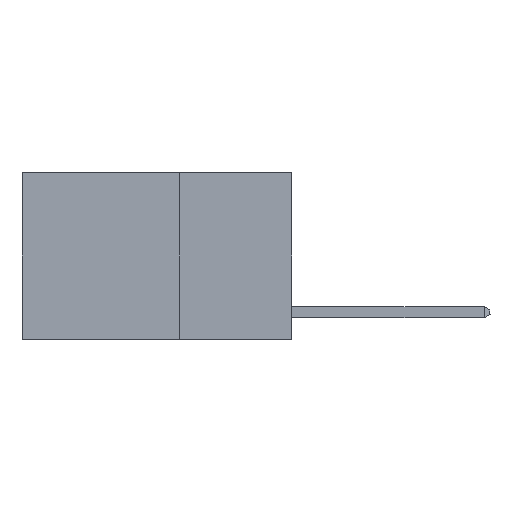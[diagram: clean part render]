
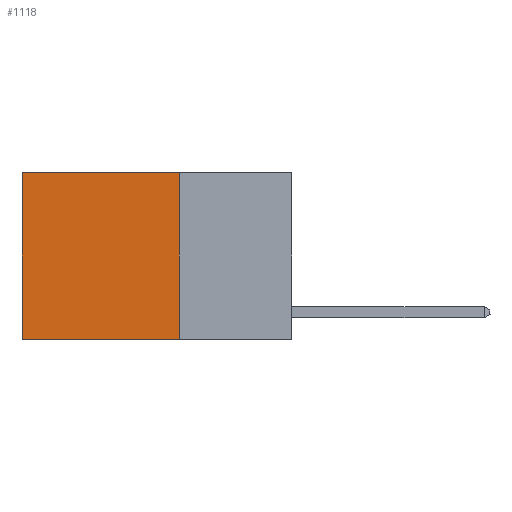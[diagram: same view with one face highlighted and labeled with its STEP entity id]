
A CAD part, left-side view. The second image highlights one B-rep face of the part: STEP entity #1118.
In plain terms, the highlighted planar face has unit normal (-1, 0, 0).
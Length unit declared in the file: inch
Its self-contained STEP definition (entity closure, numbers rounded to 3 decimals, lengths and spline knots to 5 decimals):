
#65 = EDGE_CURVE ( 'NONE', #1723, #16743, #3943, .T. ) ;
#188 = LINE ( 'NONE', #7931, #7186 ) ;
#267 = CARTESIAN_POINT ( 'NONE',  ( 0.2625, 0.25, 0. ) ) ;
#1118 = ADVANCED_FACE ( 'NONE', ( #10005 ), #15180, .F. ) ;
#1376 = CARTESIAN_POINT ( 'NONE',  ( 0.2625, 0.6, 0. ) ) ;
#1678 = EDGE_CURVE ( 'NONE', #10266, #13457, #188, .T. ) ;
#1723 = VERTEX_POINT ( 'NONE', #267 ) ;
#1963 = DIRECTION ( 'NONE',  ( 0., 0., -1. ) ) ;
#2566 = DIRECTION ( 'NONE',  ( 0., 0., -1. ) ) ;
#3414 = LINE ( 'NONE', #11212, #5023 ) ;
#3518 = VECTOR ( 'NONE', #5572, 39.37008 ) ;
#3548 = CARTESIAN_POINT ( 'NONE',  ( 0.2625, 0.25, 0. ) ) ;
#3653 = ORIENTED_EDGE ( 'NONE', *, *, #6011, .F. ) ;
#3943 = LINE ( 'NONE', #8030, #3518 ) ;
#5023 = VECTOR ( 'NONE', #1963, 39.37008 ) ;
#5216 = LINE ( 'NONE', #1376, #8983 ) ;
#5572 = DIRECTION ( 'NONE',  ( 0., 1., 0. ) ) ;
#6011 = EDGE_CURVE ( 'NONE', #1723, #10266, #3414, .T. ) ;
#6950 = AXIS2_PLACEMENT_3D ( 'NONE', #3548, #8737, #16693 ) ;
#7186 = VECTOR ( 'NONE', #15909, 39.37008 ) ;
#7789 = EDGE_LOOP ( 'NONE', ( #13212, #16571, #3653, #11039 ) ) ;
#7931 = CARTESIAN_POINT ( 'NONE',  ( 0.2625, 0.25, -0.37 ) ) ;
#8030 = CARTESIAN_POINT ( 'NONE',  ( 0.2625, 0.25, 0. ) ) ;
#8648 = CARTESIAN_POINT ( 'NONE',  ( 0.2625, 0.6, 0. ) ) ;
#8737 = DIRECTION ( 'NONE',  ( 1., 0., 0. ) ) ;
#8983 = VECTOR ( 'NONE', #2566, 39.37008 ) ;
#10005 = FACE_OUTER_BOUND ( 'NONE', #7789, .T. ) ;
#10266 = VERTEX_POINT ( 'NONE', #12816 ) ;
#10996 = CARTESIAN_POINT ( 'NONE',  ( 0.2625, 0.6, -0.37 ) ) ;
#11039 = ORIENTED_EDGE ( 'NONE', *, *, #65, .T. ) ;
#11212 = CARTESIAN_POINT ( 'NONE',  ( 0.2625, 0.25, 0. ) ) ;
#12816 = CARTESIAN_POINT ( 'NONE',  ( 0.2625, 0.25, -0.37 ) ) ;
#13212 = ORIENTED_EDGE ( 'NONE', *, *, #13666, .T. ) ;
#13457 = VERTEX_POINT ( 'NONE', #10996 ) ;
#13666 = EDGE_CURVE ( 'NONE', #16743, #13457, #5216, .T. ) ;
#15180 = PLANE ( 'NONE',  #6950 ) ;
#15909 = DIRECTION ( 'NONE',  ( 0., 1., 0. ) ) ;
#16571 = ORIENTED_EDGE ( 'NONE', *, *, #1678, .F. ) ;
#16693 = DIRECTION ( 'NONE',  ( 0., 0., -1. ) ) ;
#16743 = VERTEX_POINT ( 'NONE', #8648 ) ;
